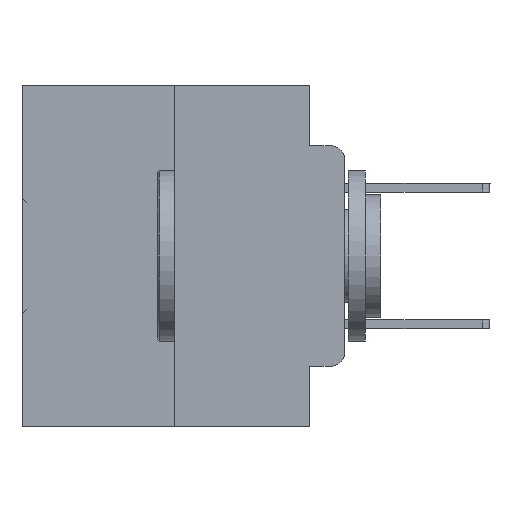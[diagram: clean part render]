
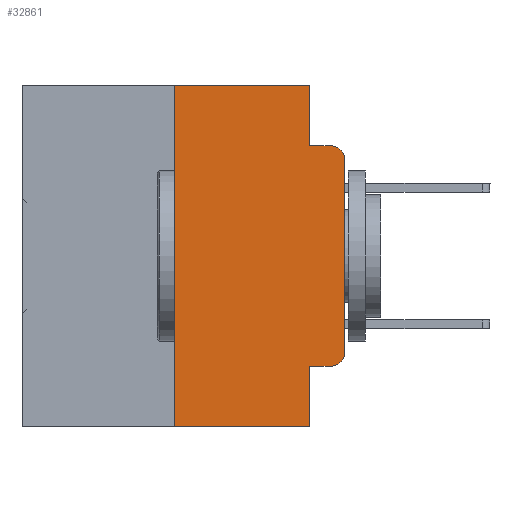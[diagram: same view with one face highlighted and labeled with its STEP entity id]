
A CAD part, left-side view. The second image highlights one B-rep face of the part: STEP entity #32861.
In plain terms, the highlighted planar face has unit normal (-1, 0, 0).
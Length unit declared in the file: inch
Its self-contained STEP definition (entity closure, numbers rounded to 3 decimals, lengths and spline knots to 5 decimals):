
#9 = PLANE ( 'NONE',  #27654 ) ;
#70 = CARTESIAN_POINT ( 'NONE',  ( 0., 0.25, -0.5 ) ) ;
#702 = CARTESIAN_POINT ( 'NONE',  ( 0., 0.02, -0.4115 ) ) ;
#753 = FACE_OUTER_BOUND ( 'NONE', #7690, .T. ) ;
#816 = ORIENTED_EDGE ( 'NONE', *, *, #11117, .T. ) ;
#1007 = LINE ( 'NONE', #27907, #14373 ) ;
#1191 = CARTESIAN_POINT ( 'NONE',  ( 0., 0.051, -0.0885 ) ) ;
#1689 = DIRECTION ( 'NONE',  ( 0., 0., 1. ) ) ;
#1917 = CARTESIAN_POINT ( 'NONE',  ( 0., 0.25, 0. ) ) ;
#2716 = ORIENTED_EDGE ( 'NONE', *, *, #6003, .T. ) ;
#3238 = EDGE_CURVE ( 'NONE', #18407, #10389, #20168, .T. ) ;
#3322 = ORIENTED_EDGE ( 'NONE', *, *, #33298, .T. ) ;
#4250 = CARTESIAN_POINT ( 'NONE',  ( 0., 0., -0.1085 ) ) ;
#4404 = CARTESIAN_POINT ( 'NONE',  ( 0., 0.02, -0.3915 ) ) ;
#5557 = CARTESIAN_POINT ( 'NONE',  ( 0., 0.473, 0. ) ) ;
#6003 = EDGE_CURVE ( 'NONE', #21662, #28182, #30892, .T. ) ;
#6302 = CARTESIAN_POINT ( 'NONE',  ( 0., 0.051, -0.5 ) ) ;
#6995 = DIRECTION ( 'NONE',  ( -1., 0., 0. ) ) ;
#7690 = EDGE_LOOP ( 'NONE', ( #816, #24586, #13776, #16723, #16552, #9770, #2716, #19234, #33456, #3322 ) ) ;
#8387 = LINE ( 'NONE', #5557, #28451 ) ;
#8422 = CARTESIAN_POINT ( 'NONE',  ( 0., 0.051, -0.4115 ) ) ;
#8660 = DIRECTION ( 'NONE',  ( 0., 0., -1. ) ) ;
#8729 = VECTOR ( 'NONE', #33197, 39.37008 ) ;
#8788 = CARTESIAN_POINT ( 'NONE',  ( 0., 0.051, 0. ) ) ;
#9150 = VERTEX_POINT ( 'NONE', #23144 ) ;
#9533 = DIRECTION ( 'NONE',  ( 0., 0., -1. ) ) ;
#9770 = ORIENTED_EDGE ( 'NONE', *, *, #13526, .F. ) ;
#9963 = EDGE_CURVE ( 'NONE', #20000, #32493, #18007, .T. ) ;
#10389 = VERTEX_POINT ( 'NONE', #702 ) ;
#10812 = CARTESIAN_POINT ( 'NONE',  ( 0., 0.473, 0. ) ) ;
#11117 = EDGE_CURVE ( 'NONE', #9150, #23918, #16670, .T. ) ;
#11243 = VECTOR ( 'NONE', #30320, 39.37008 ) ;
#11671 = CARTESIAN_POINT ( 'NONE',  ( 0., 0.051, -0.4115 ) ) ;
#11749 = AXIS2_PLACEMENT_3D ( 'NONE', #28358, #6995, #15090 ) ;
#11858 = CARTESIAN_POINT ( 'NONE',  ( 0., 0.051, 0. ) ) ;
#13392 = VERTEX_POINT ( 'NONE', #27747 ) ;
#13526 = EDGE_CURVE ( 'NONE', #21662, #13392, #17822, .T. ) ;
#13776 = ORIENTED_EDGE ( 'NONE', *, *, #33586, .F. ) ;
#14373 = VECTOR ( 'NONE', #14595, 39.37008 ) ;
#14595 = DIRECTION ( 'NONE',  ( 0., 0., -1. ) ) ;
#15090 = DIRECTION ( 'NONE',  ( 0., 0., -1. ) ) ;
#15360 = EDGE_CURVE ( 'NONE', #18407, #28182, #1007, .T. ) ;
#16552 = ORIENTED_EDGE ( 'NONE', *, *, #30566, .F. ) ;
#16609 = EDGE_CURVE ( 'NONE', #23918, #18537, #25982, .T. ) ;
#16670 = LINE ( 'NONE', #19434, #11243 ) ;
#16723 = ORIENTED_EDGE ( 'NONE', *, *, #9963, .F. ) ;
#17005 = VECTOR ( 'NONE', #1689, 39.37008 ) ;
#17016 = CIRCLE ( 'NONE', #32347, 0.02 ) ;
#17306 = VECTOR ( 'NONE', #27468, 39.37008 ) ;
#17822 = LINE ( 'NONE', #1917, #17005 ) ;
#18007 = LINE ( 'NONE', #8788, #30576 ) ;
#18407 = VERTEX_POINT ( 'NONE', #11671 ) ;
#18537 = VERTEX_POINT ( 'NONE', #33839 ) ;
#19234 = ORIENTED_EDGE ( 'NONE', *, *, #15360, .F. ) ;
#19434 = CARTESIAN_POINT ( 'NONE',  ( 0., 0., 0. ) ) ;
#20000 = VERTEX_POINT ( 'NONE', #11858 ) ;
#20168 = LINE ( 'NONE', #8422, #17306 ) ;
#21662 = VERTEX_POINT ( 'NONE', #70 ) ;
#23144 = CARTESIAN_POINT ( 'NONE',  ( 0., 0., -0.3915 ) ) ;
#23918 = VERTEX_POINT ( 'NONE', #4250 ) ;
#24073 = VECTOR ( 'NONE', #24332, 39.37008 ) ;
#24332 = DIRECTION ( 'NONE',  ( 0., -1., 0. ) ) ;
#24586 = ORIENTED_EDGE ( 'NONE', *, *, #16609, .T. ) ;
#25335 = LINE ( 'NONE', #26940, #24073 ) ;
#25982 = CIRCLE ( 'NONE', #11749, 0.02 ) ;
#26940 = CARTESIAN_POINT ( 'NONE',  ( 0., 0.051, -0.0885 ) ) ;
#27468 = DIRECTION ( 'NONE',  ( 0., -1., 0. ) ) ;
#27654 = AXIS2_PLACEMENT_3D ( 'NONE', #10812, #29411, #31896 ) ;
#27747 = CARTESIAN_POINT ( 'NONE',  ( 0., 0.25, 0. ) ) ;
#27907 = CARTESIAN_POINT ( 'NONE',  ( 0., 0.051, 0. ) ) ;
#28182 = VERTEX_POINT ( 'NONE', #6302 ) ;
#28358 = CARTESIAN_POINT ( 'NONE',  ( 0., 0.02, -0.1085 ) ) ;
#28451 = VECTOR ( 'NONE', #34509, 39.37008 ) ;
#29411 = DIRECTION ( 'NONE',  ( 1., 0., 0. ) ) ;
#30320 = DIRECTION ( 'NONE',  ( 0., 0., 1. ) ) ;
#30529 = CARTESIAN_POINT ( 'NONE',  ( 0., 0.473, -0.5 ) ) ;
#30566 = EDGE_CURVE ( 'NONE', #13392, #20000, #8387, .T. ) ;
#30576 = VECTOR ( 'NONE', #8660, 39.37008 ) ;
#30892 = LINE ( 'NONE', #30529, #8729 ) ;
#31896 = DIRECTION ( 'NONE',  ( 0., 0., -1. ) ) ;
#32347 = AXIS2_PLACEMENT_3D ( 'NONE', #4404, #33598, #9533 ) ;
#32493 = VERTEX_POINT ( 'NONE', #1191 ) ;
#32861 = ADVANCED_FACE ( 'NONE', ( #753 ), #9, .F. ) ;
#33197 = DIRECTION ( 'NONE',  ( 0., -1., 0. ) ) ;
#33298 = EDGE_CURVE ( 'NONE', #10389, #9150, #17016, .T. ) ;
#33456 = ORIENTED_EDGE ( 'NONE', *, *, #3238, .T. ) ;
#33586 = EDGE_CURVE ( 'NONE', #32493, #18537, #25335, .T. ) ;
#33598 = DIRECTION ( 'NONE',  ( -1., 0., 0. ) ) ;
#33839 = CARTESIAN_POINT ( 'NONE',  ( 0., 0.02, -0.0885 ) ) ;
#34509 = DIRECTION ( 'NONE',  ( 0., -1., 0. ) ) ;
